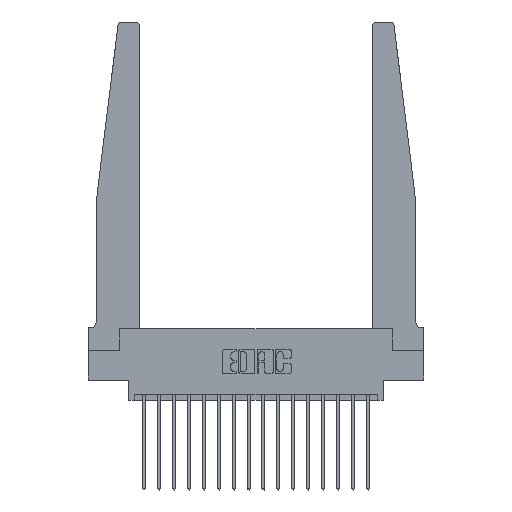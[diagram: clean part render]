
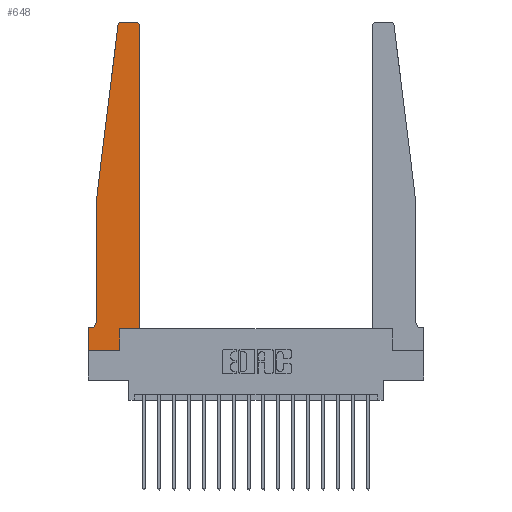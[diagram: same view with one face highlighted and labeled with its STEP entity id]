
A CAD part, top view. The second image highlights one B-rep face of the part: STEP entity #648.
In plain terms, the highlighted planar face has unit normal (0, 0, 1).
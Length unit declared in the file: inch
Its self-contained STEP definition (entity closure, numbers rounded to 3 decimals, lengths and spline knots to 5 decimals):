
#143 = LINE ( 'NONE', #4559, #2662 ) ;
#446 = AXIS2_PLACEMENT_3D ( 'NONE', #15284, #6283, #1782 ) ;
#515 = CARTESIAN_POINT ( 'NONE',  ( 0.425, 0.18, 0.37 ) ) ;
#648 = ADVANCED_FACE ( 'NONE', ( #11588 ), #8861, .T. ) ;
#731 = LINE ( 'NONE', #17907, #9300 ) ;
#1149 = CIRCLE ( 'NONE', #3352, 0.03 ) ;
#1220 = DIRECTION ( 'NONE',  ( 0., 0., 1. ) ) ;
#1782 = DIRECTION ( 'NONE',  ( 1., 0., 0. ) ) ;
#2101 = DIRECTION ( 'NONE',  ( 0., -1., 0. ) ) ;
#2134 = VERTEX_POINT ( 'NONE', #7517 ) ;
#2662 = VECTOR ( 'NONE', #16676, 39.37008 ) ;
#2826 = VERTEX_POINT ( 'NONE', #17794 ) ;
#2953 = EDGE_CURVE ( 'NONE', #12818, #4803, #7308, .T. ) ;
#3101 = VECTOR ( 'NONE', #15919, 39.37008 ) ;
#3352 = AXIS2_PLACEMENT_3D ( 'NONE', #14096, #5088, #15537 ) ;
#3614 = EDGE_CURVE ( 'NONE', #4954, #12884, #14315, .T. ) ;
#3629 = ORIENTED_EDGE ( 'NONE', *, *, #3614, .T. ) ;
#3727 = EDGE_CURVE ( 'NONE', #17302, #14785, #16213, .T. ) ;
#4027 = VECTOR ( 'NONE', #8747, 39.37008 ) ;
#4155 = CARTESIAN_POINT ( 'NONE',  ( 0., 0.1875, 0.37 ) ) ;
#4159 = LINE ( 'NONE', #8575, #11426 ) ;
#4325 = ORIENTED_EDGE ( 'NONE', *, *, #5757, .T. ) ;
#4431 = DIRECTION ( 'NONE',  ( -1., 0., 0. ) ) ;
#4559 = CARTESIAN_POINT ( 'NONE',  ( 0.425, 0.18, 0.37 ) ) ;
#4803 = VERTEX_POINT ( 'NONE', #15709 ) ;
#4921 = ORIENTED_EDGE ( 'NONE', *, *, #5960, .T. ) ;
#4954 = VERTEX_POINT ( 'NONE', #10317 ) ;
#5088 = DIRECTION ( 'NONE',  ( 0., 0., 1. ) ) ;
#5757 = EDGE_CURVE ( 'NONE', #4803, #2826, #13734, .T. ) ;
#5960 = EDGE_CURVE ( 'NONE', #12884, #17302, #16618, .T. ) ;
#6136 = ORIENTED_EDGE ( 'NONE', *, *, #8657, .T. ) ;
#6283 = DIRECTION ( 'NONE',  ( 0., 0., 1. ) ) ;
#6286 = DIRECTION ( 'NONE',  ( -1., 0., 0. ) ) ;
#6400 = VECTOR ( 'NONE', #2101, 39.37008 ) ;
#6482 = ORIENTED_EDGE ( 'NONE', *, *, #12218, .T. ) ;
#6674 = ORIENTED_EDGE ( 'NONE', *, *, #9805, .T. ) ;
#7117 = DIRECTION ( 'NONE',  ( 0., 0., -1. ) ) ;
#7193 = DIRECTION ( 'NONE',  ( 1., 0., 0. ) ) ;
#7308 = CIRCLE ( 'NONE', #9179, 0.05 ) ;
#7379 = VECTOR ( 'NONE', #17883, 39.37008 ) ;
#7517 = CARTESIAN_POINT ( 'NONE',  ( 0.395, 2.75, 0.37 ) ) ;
#7729 = VERTEX_POINT ( 'NONE', #15409 ) ;
#7964 = VERTEX_POINT ( 'NONE', #18919 ) ;
#8093 = DIRECTION ( 'NONE',  ( -0.122, -0.992, 0. ) ) ;
#8502 = CARTESIAN_POINT ( 'NONE',  ( 0.015, 0.2375, 0.37 ) ) ;
#8575 = CARTESIAN_POINT ( 'NONE',  ( 0.065, 1.25, 0.37 ) ) ;
#8592 = DIRECTION ( 'NONE',  ( -1., 0., 0. ) ) ;
#8657 = EDGE_CURVE ( 'NONE', #10712, #2134, #1149, .T. ) ;
#8747 = DIRECTION ( 'NONE',  ( 1., 0., 0. ) ) ;
#8804 = CARTESIAN_POINT ( 'NONE',  ( 0.24675, 2.72367, 0.37 ) ) ;
#8810 = CARTESIAN_POINT ( 'NONE',  ( 0.425, 0.18, 0.37 ) ) ;
#8861 = PLANE ( 'NONE',  #9154 ) ;
#8910 = CIRCLE ( 'NONE', #446, 0.03 ) ;
#9154 = AXIS2_PLACEMENT_3D ( 'NONE', #4155, #1220, #7193 ) ;
#9179 = AXIS2_PLACEMENT_3D ( 'NONE', #8502, #7117, #8592 ) ;
#9300 = VECTOR ( 'NONE', #4431, 39.37008 ) ;
#9541 = LINE ( 'NONE', #15491, #16362 ) ;
#9805 = EDGE_CURVE ( 'NONE', #2134, #7729, #731, .T. ) ;
#10317 = CARTESIAN_POINT ( 'NONE',  ( 0., 0., 0.37 ) ) ;
#10712 = VERTEX_POINT ( 'NONE', #12089 ) ;
#11146 = ORIENTED_EDGE ( 'NONE', *, *, #13233, .T. ) ;
#11152 = CARTESIAN_POINT ( 'NONE',  ( 0.2605, 0.18, 0.37 ) ) ;
#11277 = ORIENTED_EDGE ( 'NONE', *, *, #11712, .T. ) ;
#11426 = VECTOR ( 'NONE', #11593, 39.37008 ) ;
#11447 = VECTOR ( 'NONE', #6286, 39.37008 ) ;
#11588 = FACE_OUTER_BOUND ( 'NONE', #17895, .T. ) ;
#11593 = DIRECTION ( 'NONE',  ( 0., -1., 0. ) ) ;
#11712 = EDGE_CURVE ( 'NONE', #14785, #10712, #143, .T. ) ;
#11950 = CARTESIAN_POINT ( 'NONE',  ( 0.2605, 0.18, 0.37 ) ) ;
#12089 = CARTESIAN_POINT ( 'NONE',  ( 0.425, 2.72, 0.37 ) ) ;
#12098 = EDGE_CURVE ( 'NONE', #7729, #15113, #8910, .T. ) ;
#12218 = EDGE_CURVE ( 'NONE', #2826, #4954, #16650, .T. ) ;
#12460 = ORIENTED_EDGE ( 'NONE', *, *, #2953, .T. ) ;
#12818 = VERTEX_POINT ( 'NONE', #19206 ) ;
#12884 = VERTEX_POINT ( 'NONE', #13088 ) ;
#13088 = CARTESIAN_POINT ( 'NONE',  ( 0.2605, 0., 0.37 ) ) ;
#13233 = EDGE_CURVE ( 'NONE', #7964, #12818, #4159, .T. ) ;
#13734 = LINE ( 'NONE', #18410, #11447 ) ;
#14065 = ORIENTED_EDGE ( 'NONE', *, *, #18112, .T. ) ;
#14096 = CARTESIAN_POINT ( 'NONE',  ( 0.395, 2.72, 0.37 ) ) ;
#14315 = LINE ( 'NONE', #14408, #4027 ) ;
#14332 = ORIENTED_EDGE ( 'NONE', *, *, #12098, .T. ) ;
#14408 = CARTESIAN_POINT ( 'NONE',  ( 0., 0., 0.37 ) ) ;
#14785 = VERTEX_POINT ( 'NONE', #515 ) ;
#15113 = VERTEX_POINT ( 'NONE', #8804 ) ;
#15284 = CARTESIAN_POINT ( 'NONE',  ( 0.27653, 2.72, 0.37 ) ) ;
#15409 = CARTESIAN_POINT ( 'NONE',  ( 0.27653, 2.75, 0.37 ) ) ;
#15491 = CARTESIAN_POINT ( 'NONE',  ( 0.065, 1.25, 0.37 ) ) ;
#15537 = DIRECTION ( 'NONE',  ( 1., 0., 0. ) ) ;
#15709 = CARTESIAN_POINT ( 'NONE',  ( 0.015, 0.1875, 0.37 ) ) ;
#15890 = ORIENTED_EDGE ( 'NONE', *, *, #3727, .T. ) ;
#15919 = DIRECTION ( 'NONE',  ( 1., 0., 0. ) ) ;
#16213 = LINE ( 'NONE', #8810, #3101 ) ;
#16362 = VECTOR ( 'NONE', #8093, 39.37008 ) ;
#16618 = LINE ( 'NONE', #11950, #7379 ) ;
#16650 = LINE ( 'NONE', #18506, #6400 ) ;
#16676 = DIRECTION ( 'NONE',  ( 0., 1., 0. ) ) ;
#17302 = VERTEX_POINT ( 'NONE', #11152 ) ;
#17794 = CARTESIAN_POINT ( 'NONE',  ( 0., 0.1875, 0.37 ) ) ;
#17883 = DIRECTION ( 'NONE',  ( 0., 1., 0. ) ) ;
#17895 = EDGE_LOOP ( 'NONE', ( #6674, #14332, #14065, #11146, #12460, #4325, #6482, #3629, #4921, #15890, #11277, #6136 ) ) ;
#17907 = CARTESIAN_POINT ( 'NONE',  ( 0.25, 2.75, 0.37 ) ) ;
#18112 = EDGE_CURVE ( 'NONE', #15113, #7964, #9541, .T. ) ;
#18410 = CARTESIAN_POINT ( 'NONE',  ( 0.065, 0.1875, 0.37 ) ) ;
#18506 = CARTESIAN_POINT ( 'NONE',  ( 0., 0., 0.37 ) ) ;
#18919 = CARTESIAN_POINT ( 'NONE',  ( 0.065, 1.25, 0.37 ) ) ;
#19206 = CARTESIAN_POINT ( 'NONE',  ( 0.065, 0.2375, 0.37 ) ) ;
